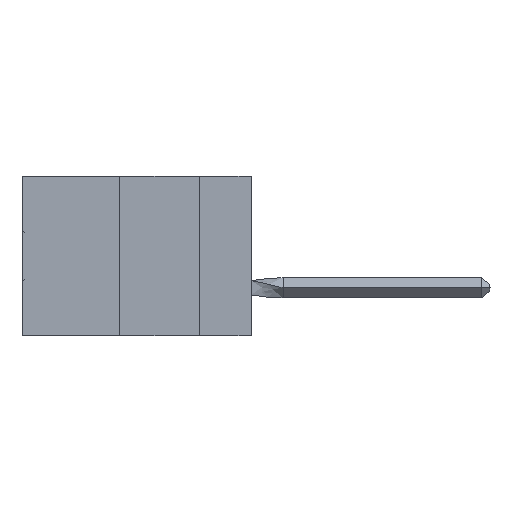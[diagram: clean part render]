
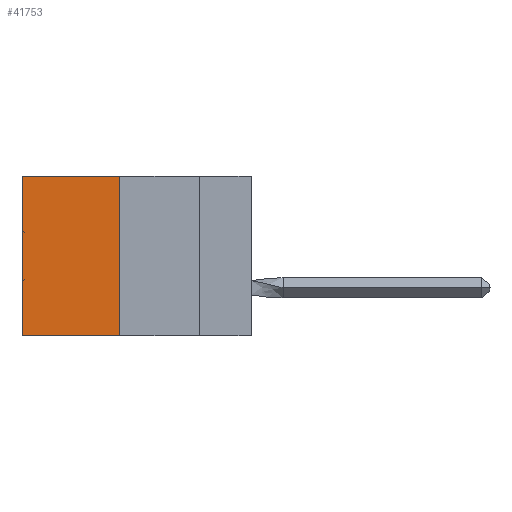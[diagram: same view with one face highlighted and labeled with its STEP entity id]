
A CAD part, left-side view. The second image highlights one B-rep face of the part: STEP entity #41753.
In plain terms, the highlighted planar face has unit normal (-1, 0, 0).
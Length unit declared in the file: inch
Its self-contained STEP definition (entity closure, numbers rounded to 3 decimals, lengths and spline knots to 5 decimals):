
#290 = FACE_OUTER_BOUND ( 'NONE', #38466, .T. ) ;
#1276 = EDGE_CURVE ( 'NONE', #25956, #48167, #26824, .T. ) ;
#2047 = LINE ( 'NONE', #47901, #33575 ) ;
#2835 = DIRECTION ( 'NONE',  ( 0., 1., 0. ) ) ;
#3322 = DIRECTION ( 'NONE',  ( 0., 0., -1. ) ) ;
#3381 = DIRECTION ( 'NONE',  ( 1., 0., 0. ) ) ;
#6548 = LINE ( 'NONE', #32386, #45949 ) ;
#6590 = CARTESIAN_POINT ( 'NONE',  ( 0.305, 0.72, 0. ) ) ;
#10047 = LINE ( 'NONE', #46115, #21138 ) ;
#10984 = ORIENTED_EDGE ( 'NONE', *, *, #1276, .F. ) ;
#11670 = DIRECTION ( 'NONE',  ( 0., 1., 0. ) ) ;
#14473 = CARTESIAN_POINT ( 'NONE',  ( 0.305, 0.413, 0. ) ) ;
#14991 = EDGE_CURVE ( 'NONE', #36297, #19476, #6548, .T. ) ;
#17344 = ORIENTED_EDGE ( 'NONE', *, *, #43217, .T. ) ;
#19476 = VERTEX_POINT ( 'NONE', #6590 ) ;
#20424 = CARTESIAN_POINT ( 'NONE',  ( 0.305, 0.413, -0.5 ) ) ;
#20536 = ORIENTED_EDGE ( 'NONE', *, *, #42411, .F. ) ;
#21138 = VECTOR ( 'NONE', #3322, 39.37008 ) ;
#24356 = AXIS2_PLACEMENT_3D ( 'NONE', #20424, #3381, #24595 ) ;
#24595 = DIRECTION ( 'NONE',  ( 0., 0., -1. ) ) ;
#24959 = CARTESIAN_POINT ( 'NONE',  ( 0.305, 0.413, -0.5 ) ) ;
#25956 = VERTEX_POINT ( 'NONE', #47292 ) ;
#26824 = LINE ( 'NONE', #24959, #53901 ) ;
#32386 = CARTESIAN_POINT ( 'NONE',  ( 0.305, 0.413, 0. ) ) ;
#32599 = PLANE ( 'NONE',  #24356 ) ;
#33575 = VECTOR ( 'NONE', #43102, 39.37008 ) ;
#36297 = VERTEX_POINT ( 'NONE', #14473 ) ;
#38466 = EDGE_LOOP ( 'NONE', ( #17344, #10984, #20536, #54115 ) ) ;
#41753 = ADVANCED_FACE ( 'NONE', ( #290 ), #32599, .F. ) ;
#42411 = EDGE_CURVE ( 'NONE', #36297, #25956, #10047, .T. ) ;
#43102 = DIRECTION ( 'NONE',  ( 0., 0., -1. ) ) ;
#43217 = EDGE_CURVE ( 'NONE', #19476, #48167, #2047, .T. ) ;
#45756 = CARTESIAN_POINT ( 'NONE',  ( 0.305, 0.72, -0.5 ) ) ;
#45949 = VECTOR ( 'NONE', #2835, 39.37008 ) ;
#46115 = CARTESIAN_POINT ( 'NONE',  ( 0.305, 0.413, -0.5 ) ) ;
#47292 = CARTESIAN_POINT ( 'NONE',  ( 0.305, 0.413, -0.5 ) ) ;
#47901 = CARTESIAN_POINT ( 'NONE',  ( 0.305, 0.72, -0.5 ) ) ;
#48167 = VERTEX_POINT ( 'NONE', #45756 ) ;
#53901 = VECTOR ( 'NONE', #11670, 39.37008 ) ;
#54115 = ORIENTED_EDGE ( 'NONE', *, *, #14991, .T. ) ;
